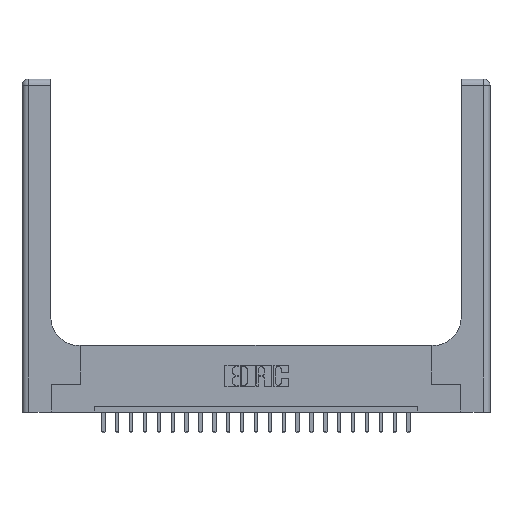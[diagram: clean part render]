
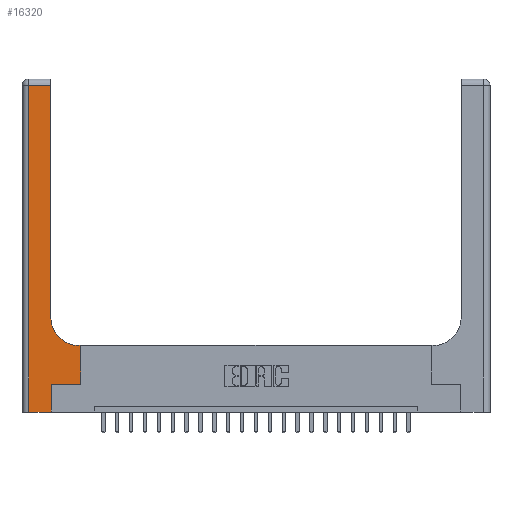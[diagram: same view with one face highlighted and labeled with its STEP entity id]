
A CAD part, top view. The second image highlights one B-rep face of the part: STEP entity #16320.
In plain terms, the highlighted planar face has unit normal (0, 0, 1).
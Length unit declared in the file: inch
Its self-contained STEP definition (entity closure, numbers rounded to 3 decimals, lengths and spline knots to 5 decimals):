
#38 = ORIENTED_EDGE ( 'NONE', *, *, #6949, .T. ) ;
#226 = EDGE_CURVE ( 'NONE', #21581, #2423, #9532, .T. ) ;
#572 = LINE ( 'NONE', #10225, #19027 ) ;
#825 = DIRECTION ( 'NONE',  ( 0., 1., 0. ) ) ;
#1750 = CIRCLE ( 'NONE', #18180, 0.25 ) ;
#2215 = EDGE_CURVE ( 'NONE', #5233, #14062, #8634, .T. ) ;
#2266 = CARTESIAN_POINT ( 'NONE',  ( 0.528, 0.6, 0.37 ) ) ;
#2423 = VERTEX_POINT ( 'NONE', #11296 ) ;
#2434 = VERTEX_POINT ( 'NONE', #12946 ) ;
#2819 = ORIENTED_EDGE ( 'NONE', *, *, #12035, .T. ) ;
#3361 = CARTESIAN_POINT ( 'NONE',  ( 0., 3., 0.37 ) ) ;
#3602 = DIRECTION ( 'NONE',  ( 0., 1., 0. ) ) ;
#3802 = ORIENTED_EDGE ( 'NONE', *, *, #21842, .T. ) ;
#3948 = CARTESIAN_POINT ( 'NONE',  ( 0.265, 0.25, 0.37 ) ) ;
#3960 = EDGE_CURVE ( 'NONE', #12577, #5233, #11264, .T. ) ;
#4408 = VERTEX_POINT ( 'NONE', #19712 ) ;
#4414 = VERTEX_POINT ( 'NONE', #7794 ) ;
#4893 = LINE ( 'NONE', #12018, #16146 ) ;
#4953 = VECTOR ( 'NONE', #825, 39.37008 ) ;
#5233 = VERTEX_POINT ( 'NONE', #19701 ) ;
#5627 = ORIENTED_EDGE ( 'NONE', *, *, #6920, .T. ) ;
#6042 = LINE ( 'NONE', #7939, #4953 ) ;
#6436 = FACE_OUTER_BOUND ( 'NONE', #16737, .T. ) ;
#6707 = CARTESIAN_POINT ( 'NONE',  ( 0.06, 0., 0.37 ) ) ;
#6920 = EDGE_CURVE ( 'NONE', #2423, #4414, #1750, .T. ) ;
#6949 = EDGE_CURVE ( 'NONE', #4414, #15934, #6042, .T. ) ;
#7438 = ORIENTED_EDGE ( 'NONE', *, *, #8160, .T. ) ;
#7728 = LINE ( 'NONE', #20207, #8265 ) ;
#7794 = CARTESIAN_POINT ( 'NONE',  ( 0.26, 0.85, 0.37 ) ) ;
#7939 = CARTESIAN_POINT ( 'NONE',  ( 0.26, 3., 0.37 ) ) ;
#8160 = EDGE_CURVE ( 'NONE', #4408, #12577, #14019, .T. ) ;
#8260 = ORIENTED_EDGE ( 'NONE', *, *, #2215, .T. ) ;
#8265 = VECTOR ( 'NONE', #8289, 39.37008 ) ;
#8289 = DIRECTION ( 'NONE',  ( 0., 1., 0. ) ) ;
#8634 = LINE ( 'NONE', #19148, #12374 ) ;
#9532 = LINE ( 'NONE', #22020, #16754 ) ;
#10225 = CARTESIAN_POINT ( 'NONE',  ( 0., 2.94, 0.37 ) ) ;
#10705 = ORIENTED_EDGE ( 'NONE', *, *, #3960, .T. ) ;
#10982 = AXIS2_PLACEMENT_3D ( 'NONE', #3361, #17053, #13672 ) ;
#11264 = LINE ( 'NONE', #21990, #13929 ) ;
#11296 = CARTESIAN_POINT ( 'NONE',  ( 0.51, 0.6, 0.37 ) ) ;
#12018 = CARTESIAN_POINT ( 'NONE',  ( 0.265, 0.25, 0.37 ) ) ;
#12035 = EDGE_CURVE ( 'NONE', #14062, #2434, #4893, .T. ) ;
#12374 = VECTOR ( 'NONE', #3602, 39.37008 ) ;
#12577 = VERTEX_POINT ( 'NONE', #6707 ) ;
#12936 = VECTOR ( 'NONE', #19587, 39.37008 ) ;
#12946 = CARTESIAN_POINT ( 'NONE',  ( 0.528, 0.25, 0.37 ) ) ;
#13424 = DIRECTION ( 'NONE',  ( -1., 0., 0. ) ) ;
#13455 = DIRECTION ( 'NONE',  ( 1., 0., 0. ) ) ;
#13472 = DIRECTION ( 'NONE',  ( 1., 0., 0. ) ) ;
#13572 = ORIENTED_EDGE ( 'NONE', *, *, #226, .T. ) ;
#13672 = DIRECTION ( 'NONE',  ( -1., 0., 0. ) ) ;
#13754 = PLANE ( 'NONE',  #10982 ) ;
#13888 = ORIENTED_EDGE ( 'NONE', *, *, #15738, .T. ) ;
#13929 = VECTOR ( 'NONE', #13472, 39.37008 ) ;
#14019 = LINE ( 'NONE', #21179, #12936 ) ;
#14062 = VERTEX_POINT ( 'NONE', #3948 ) ;
#15738 = EDGE_CURVE ( 'NONE', #15934, #4408, #572, .T. ) ;
#15934 = VERTEX_POINT ( 'NONE', #17412 ) ;
#16146 = VECTOR ( 'NONE', #13455, 39.37008 ) ;
#16320 = ADVANCED_FACE ( 'NONE', ( #6436 ), #13754, .F. ) ;
#16737 = EDGE_LOOP ( 'NONE', ( #38, #13888, #7438, #10705, #8260, #2819, #3802, #13572, #5627 ) ) ;
#16754 = VECTOR ( 'NONE', #13424, 39.37008 ) ;
#17053 = DIRECTION ( 'NONE',  ( 0., 0., -1. ) ) ;
#17412 = CARTESIAN_POINT ( 'NONE',  ( 0.26, 2.94, 0.37 ) ) ;
#18098 = CARTESIAN_POINT ( 'NONE',  ( 0.51, 0.85, 0.37 ) ) ;
#18180 = AXIS2_PLACEMENT_3D ( 'NONE', #18098, #21589, #21303 ) ;
#18747 = DIRECTION ( 'NONE',  ( -1., 0., 0. ) ) ;
#19027 = VECTOR ( 'NONE', #18747, 39.37008 ) ;
#19148 = CARTESIAN_POINT ( 'NONE',  ( 0.265, 0., 0.37 ) ) ;
#19587 = DIRECTION ( 'NONE',  ( 0., -1., 0. ) ) ;
#19701 = CARTESIAN_POINT ( 'NONE',  ( 0.265, 0., 0.37 ) ) ;
#19712 = CARTESIAN_POINT ( 'NONE',  ( 0.06, 2.94, 0.37 ) ) ;
#20207 = CARTESIAN_POINT ( 'NONE',  ( 0.528, 0.25, 0.37 ) ) ;
#21179 = CARTESIAN_POINT ( 'NONE',  ( 0.06, 3., 0.37 ) ) ;
#21303 = DIRECTION ( 'NONE',  ( 1., 0., 0. ) ) ;
#21581 = VERTEX_POINT ( 'NONE', #2266 ) ;
#21589 = DIRECTION ( 'NONE',  ( 0., 0., -1. ) ) ;
#21842 = EDGE_CURVE ( 'NONE', #2434, #21581, #7728, .T. ) ;
#21990 = CARTESIAN_POINT ( 'NONE',  ( 0., 0., 0.37 ) ) ;
#22020 = CARTESIAN_POINT ( 'NONE',  ( 0.26, 0.6, 0.37 ) ) ;
